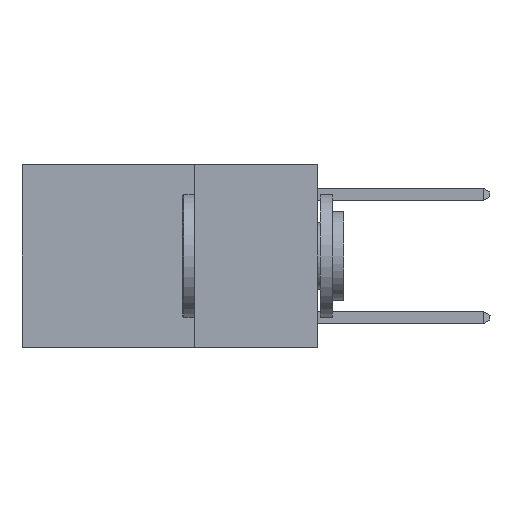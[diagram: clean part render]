
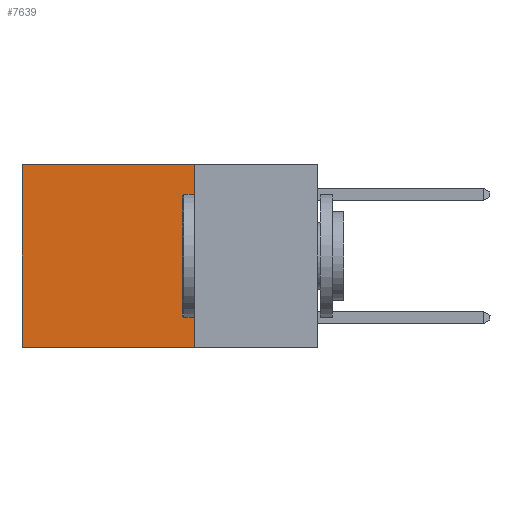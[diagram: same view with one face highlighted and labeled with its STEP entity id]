
A CAD part, left-side view. The second image highlights one B-rep face of the part: STEP entity #7639.
In plain terms, the highlighted planar face has unit normal (-1, 0, 0).
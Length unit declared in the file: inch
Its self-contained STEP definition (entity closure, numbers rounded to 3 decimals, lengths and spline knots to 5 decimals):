
#116 = LINE ( 'NONE', #4056, #5431 ) ;
#1147 = DIRECTION ( 'NONE',  ( 0., 0., -1. ) ) ;
#1294 = AXIS2_PLACEMENT_3D ( 'NONE', #5934, #13624, #1147 ) ;
#2226 = CARTESIAN_POINT ( 'NONE',  ( 0.2625, 0.25, 0. ) ) ;
#2406 = PLANE ( 'NONE',  #1294 ) ;
#2630 = VECTOR ( 'NONE', #2950, 39.37008 ) ;
#2913 = FACE_OUTER_BOUND ( 'NONE', #8547, .T. ) ;
#2950 = DIRECTION ( 'NONE',  ( 0., 0., -1. ) ) ;
#3255 = VECTOR ( 'NONE', #6095, 39.37008 ) ;
#3493 = EDGE_CURVE ( 'NONE', #8309, #14406, #5962, .T. ) ;
#4056 = CARTESIAN_POINT ( 'NONE',  ( 0.2625, 0.25, -0.37 ) ) ;
#4109 = CARTESIAN_POINT ( 'NONE',  ( 0.2625, 0.6, 0. ) ) ;
#5431 = VECTOR ( 'NONE', #7363, 39.37008 ) ;
#5460 = ORIENTED_EDGE ( 'NONE', *, *, #3493, .F. ) ;
#5934 = CARTESIAN_POINT ( 'NONE',  ( 0.2625, 0.25, 0. ) ) ;
#5962 = LINE ( 'NONE', #8324, #3255 ) ;
#6095 = DIRECTION ( 'NONE',  ( 0., 0., -1. ) ) ;
#6437 = CARTESIAN_POINT ( 'NONE',  ( 0.2625, 0.6, -0.37 ) ) ;
#7363 = DIRECTION ( 'NONE',  ( 0., 1., 0. ) ) ;
#7473 = LINE ( 'NONE', #4109, #2630 ) ;
#7639 = ADVANCED_FACE ( 'NONE', ( #2913 ), #2406, .F. ) ;
#7784 = ORIENTED_EDGE ( 'NONE', *, *, #13949, .F. ) ;
#7849 = VERTEX_POINT ( 'NONE', #6437 ) ;
#8086 = LINE ( 'NONE', #2226, #8792 ) ;
#8309 = VERTEX_POINT ( 'NONE', #10764 ) ;
#8324 = CARTESIAN_POINT ( 'NONE',  ( 0.2625, 0.25, 0. ) ) ;
#8547 = EDGE_LOOP ( 'NONE', ( #13598, #7784, #5460, #9260 ) ) ;
#8792 = VECTOR ( 'NONE', #10282, 39.37008 ) ;
#8975 = EDGE_CURVE ( 'NONE', #8309, #11905, #8086, .T. ) ;
#9260 = ORIENTED_EDGE ( 'NONE', *, *, #8975, .T. ) ;
#9403 = CARTESIAN_POINT ( 'NONE',  ( 0.2625, 0.25, -0.37 ) ) ;
#10201 = CARTESIAN_POINT ( 'NONE',  ( 0.2625, 0.6, 0. ) ) ;
#10282 = DIRECTION ( 'NONE',  ( 0., 1., 0. ) ) ;
#10764 = CARTESIAN_POINT ( 'NONE',  ( 0.2625, 0.25, 0. ) ) ;
#11655 = EDGE_CURVE ( 'NONE', #11905, #7849, #7473, .T. ) ;
#11905 = VERTEX_POINT ( 'NONE', #10201 ) ;
#13598 = ORIENTED_EDGE ( 'NONE', *, *, #11655, .T. ) ;
#13624 = DIRECTION ( 'NONE',  ( 1., 0., 0. ) ) ;
#13949 = EDGE_CURVE ( 'NONE', #14406, #7849, #116, .T. ) ;
#14406 = VERTEX_POINT ( 'NONE', #9403 ) ;
